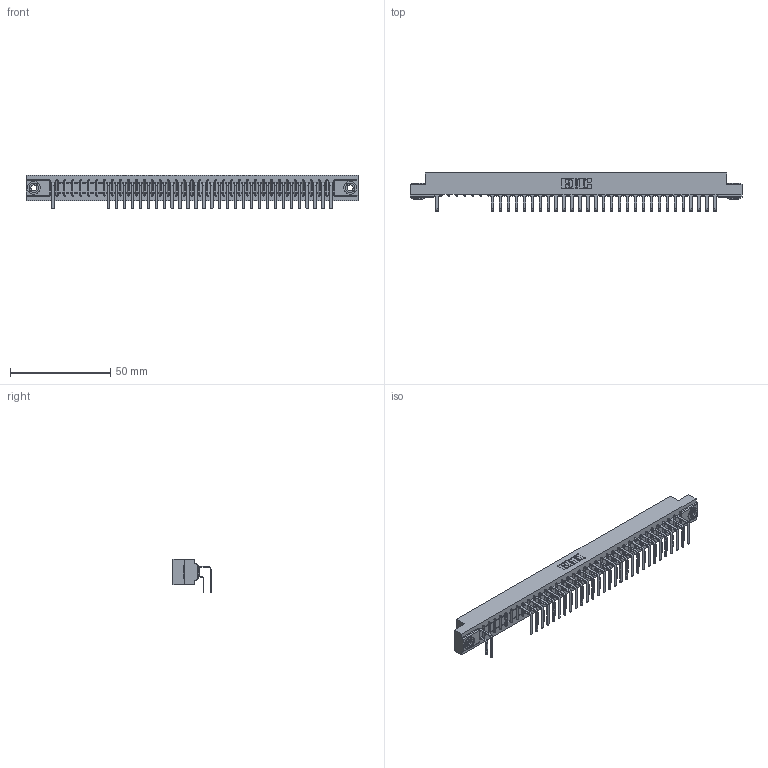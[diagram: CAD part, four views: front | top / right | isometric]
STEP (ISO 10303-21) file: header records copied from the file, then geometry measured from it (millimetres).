
FILE_DESCRIPTION (( 'STEP AP203' ), '1' );
FILE_NAME ('307-036-558-103.STEP', '2018-08-05T08:11:09', ( '' ), ( '' ), 'SwSTEP 2.0', 'SolidWorks 2016', '' );
FILE_SCHEMA (( 'CONFIG_CONTROL_DESIGN' ));
Length unit declared in the file: inch
Products named in the file (5): 307-290-001_558 - 2 (Single); 345-250-002_345-250-002-102; 307-036-558-103; 307 Part_.156 Dia Mounting Holes; 307-290-001_558 559 - 1 (Single)
Assembly tree (62 placements, depth 2):
  307-036-558-103
    307 Part_.156 Dia Mounting Holes
    307-290-001_558 559 - 1 (Single)  x29
    307-290-001_558 - 2 (Single)  x30
    345-250-002_345-250-002-102  x2
Bounding box: 165.66 x 18.96 x 16.8 mm (x, y, z)
Volume: 17669.5 mm3; surface area: 22178.4 mm2
Topology: 62 solids, 62 shells, 3287 faces, 9229 edges, 5970 vertices
Faces by surface type: plane 2119, cylinder 1086, sphere 74, cone 8
Entity records: 34850 total; most frequent: CARTESIAN_POINT 5742, ORIENTED_EDGE 5694, DIRECTION 5627, EDGE_CURVE 2847, VECTOR 2173, LINE 2173, VERTEX_POINT 1842, AXIS2_PLACEMENT_3D 1727
